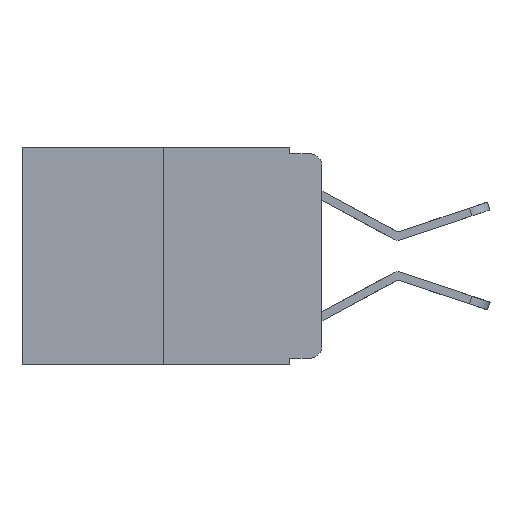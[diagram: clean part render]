
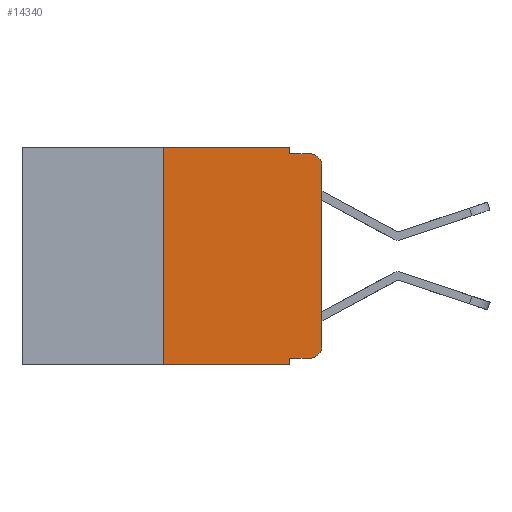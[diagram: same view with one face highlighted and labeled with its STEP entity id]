
A CAD part, left-side view. The second image highlights one B-rep face of the part: STEP entity #14340.
In plain terms, the highlighted planar face has unit normal (-1, 0, 0).
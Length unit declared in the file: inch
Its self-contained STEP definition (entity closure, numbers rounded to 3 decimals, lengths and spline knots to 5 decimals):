
#137 = EDGE_CURVE ( 'NONE', #5501, #5278, #1923, .T. ) ;
#201 = VERTEX_POINT ( 'NONE', #14986 ) ;
#341 = AXIS2_PLACEMENT_3D ( 'NONE', #1104, #17474, #738 ) ;
#385 = CARTESIAN_POINT ( 'NONE',  ( 0., 0.051, 0. ) ) ;
#483 = DIRECTION ( 'NONE',  ( 0., -1., 0. ) ) ;
#738 = DIRECTION ( 'NONE',  ( 0., 0., -1. ) ) ;
#1038 = EDGE_CURVE ( 'NONE', #21150, #1491, #20355, .T. ) ;
#1104 = CARTESIAN_POINT ( 'NONE',  ( 0., 0.02, -0.313 ) ) ;
#1224 = DIRECTION ( 'NONE',  ( 0., -1., 0. ) ) ;
#1491 = VERTEX_POINT ( 'NONE', #18278 ) ;
#1661 = ORIENTED_EDGE ( 'NONE', *, *, #14019, .F. ) ;
#1765 = ORIENTED_EDGE ( 'NONE', *, *, #2188, .T. ) ;
#1923 = LINE ( 'NONE', #18750, #6572 ) ;
#2011 = VERTEX_POINT ( 'NONE', #13185 ) ;
#2188 = EDGE_CURVE ( 'NONE', #9574, #14017, #23702, .T. ) ;
#2437 = CARTESIAN_POINT ( 'NONE',  ( 0., 0.473, 0. ) ) ;
#2446 = DIRECTION ( 'NONE',  ( 0., -1., 0. ) ) ;
#3071 = LINE ( 'NONE', #10509, #13448 ) ;
#3350 = DIRECTION ( 'NONE',  ( 0., 0., -1. ) ) ;
#3621 = CARTESIAN_POINT ( 'NONE',  ( 0., 0.25, 0. ) ) ;
#3885 = DIRECTION ( 'NONE',  ( 1., 0., 0. ) ) ;
#4738 = CARTESIAN_POINT ( 'NONE',  ( 0., 0.02, -0.03 ) ) ;
#5278 = VERTEX_POINT ( 'NONE', #6147 ) ;
#5482 = VERTEX_POINT ( 'NONE', #9174 ) ;
#5501 = VERTEX_POINT ( 'NONE', #385 ) ;
#6033 = VECTOR ( 'NONE', #2446, 39.37008 ) ;
#6147 = CARTESIAN_POINT ( 'NONE',  ( 0., 0.051, -0.01 ) ) ;
#6327 = DIRECTION ( 'NONE',  ( -1., 0., 0. ) ) ;
#6572 = VECTOR ( 'NONE', #19007, 39.37008 ) ;
#6683 = ORIENTED_EDGE ( 'NONE', *, *, #10858, .T. ) ;
#8496 = AXIS2_PLACEMENT_3D ( 'NONE', #4738, #6327, #19634 ) ;
#9174 = CARTESIAN_POINT ( 'NONE',  ( 0., 0.051, -0.333 ) ) ;
#9252 = DIRECTION ( 'NONE',  ( 0., 0., 1. ) ) ;
#9574 = VERTEX_POINT ( 'NONE', #12128 ) ;
#9754 = LINE ( 'NONE', #2437, #23325 ) ;
#10019 = LINE ( 'NONE', #18938, #6033 ) ;
#10468 = CIRCLE ( 'NONE', #341, 0.02 ) ;
#10509 = CARTESIAN_POINT ( 'NONE',  ( 0., 0.473, -0.343 ) ) ;
#10853 = ORIENTED_EDGE ( 'NONE', *, *, #15089, .F. ) ;
#10858 = EDGE_CURVE ( 'NONE', #2011, #9574, #12618, .T. ) ;
#11265 = CARTESIAN_POINT ( 'NONE',  ( 0., 0.051, -0.343 ) ) ;
#11601 = CARTESIAN_POINT ( 'NONE',  ( 0., 0.02, -0.01 ) ) ;
#12128 = CARTESIAN_POINT ( 'NONE',  ( 0., 0., -0.03 ) ) ;
#12618 = LINE ( 'NONE', #21918, #20861 ) ;
#12703 = EDGE_LOOP ( 'NONE', ( #6683, #1765, #13859, #19326, #1661, #12807, #20180, #10853, #21532, #17613 ) ) ;
#12765 = VECTOR ( 'NONE', #22784, 39.37008 ) ;
#12807 = ORIENTED_EDGE ( 'NONE', *, *, #1038, .F. ) ;
#13180 = EDGE_CURVE ( 'NONE', #5278, #14017, #23021, .T. ) ;
#13185 = CARTESIAN_POINT ( 'NONE',  ( 0., 0., -0.313 ) ) ;
#13388 = FACE_OUTER_BOUND ( 'NONE', #12703, .T. ) ;
#13448 = VECTOR ( 'NONE', #1224, 39.37008 ) ;
#13859 = ORIENTED_EDGE ( 'NONE', *, *, #13180, .F. ) ;
#14017 = VERTEX_POINT ( 'NONE', #11601 ) ;
#14019 = EDGE_CURVE ( 'NONE', #1491, #5501, #9754, .T. ) ;
#14082 = EDGE_CURVE ( 'NONE', #201, #2011, #10468, .T. ) ;
#14340 = ADVANCED_FACE ( 'NONE', ( #13388 ), #22563, .F. ) ;
#14986 = CARTESIAN_POINT ( 'NONE',  ( 0., 0.02, -0.333 ) ) ;
#15089 = EDGE_CURVE ( 'NONE', #5482, #15218, #23839, .T. ) ;
#15218 = VERTEX_POINT ( 'NONE', #11265 ) ;
#15422 = VECTOR ( 'NONE', #3350, 39.37008 ) ;
#15947 = AXIS2_PLACEMENT_3D ( 'NONE', #18886, #3885, #18759 ) ;
#16175 = CARTESIAN_POINT ( 'NONE',  ( 0., 0.051, 0. ) ) ;
#17084 = EDGE_CURVE ( 'NONE', #5482, #201, #10019, .T. ) ;
#17297 = VECTOR ( 'NONE', #9252, 39.37008 ) ;
#17302 = EDGE_CURVE ( 'NONE', #21150, #15218, #3071, .T. ) ;
#17474 = DIRECTION ( 'NONE',  ( -1., 0., 0. ) ) ;
#17613 = ORIENTED_EDGE ( 'NONE', *, *, #14082, .T. ) ;
#18278 = CARTESIAN_POINT ( 'NONE',  ( 0., 0.25, 0. ) ) ;
#18750 = CARTESIAN_POINT ( 'NONE',  ( 0., 0.051, 0. ) ) ;
#18759 = DIRECTION ( 'NONE',  ( 0., 0., -1. ) ) ;
#18886 = CARTESIAN_POINT ( 'NONE',  ( 0., 0.473, 0. ) ) ;
#18938 = CARTESIAN_POINT ( 'NONE',  ( 0., 0.051, -0.333 ) ) ;
#19007 = DIRECTION ( 'NONE',  ( 0., 0., -1. ) ) ;
#19165 = CARTESIAN_POINT ( 'NONE',  ( 0., 0.25, -0.343 ) ) ;
#19326 = ORIENTED_EDGE ( 'NONE', *, *, #137, .F. ) ;
#19634 = DIRECTION ( 'NONE',  ( 0., 0., -1. ) ) ;
#20180 = ORIENTED_EDGE ( 'NONE', *, *, #17302, .T. ) ;
#20355 = LINE ( 'NONE', #3621, #17297 ) ;
#20861 = VECTOR ( 'NONE', #23493, 39.37008 ) ;
#21150 = VERTEX_POINT ( 'NONE', #19165 ) ;
#21339 = CARTESIAN_POINT ( 'NONE',  ( 0., 0.051, -0.01 ) ) ;
#21532 = ORIENTED_EDGE ( 'NONE', *, *, #17084, .T. ) ;
#21918 = CARTESIAN_POINT ( 'NONE',  ( 0., 0., 0. ) ) ;
#22563 = PLANE ( 'NONE',  #15947 ) ;
#22784 = DIRECTION ( 'NONE',  ( 0., -1., 0. ) ) ;
#23021 = LINE ( 'NONE', #21339, #12765 ) ;
#23325 = VECTOR ( 'NONE', #483, 39.37008 ) ;
#23493 = DIRECTION ( 'NONE',  ( 0., 0., 1. ) ) ;
#23702 = CIRCLE ( 'NONE', #8496, 0.02 ) ;
#23839 = LINE ( 'NONE', #16175, #15422 ) ;
